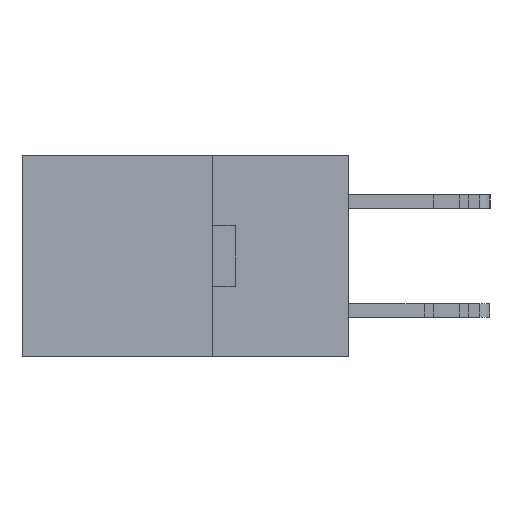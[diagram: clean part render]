
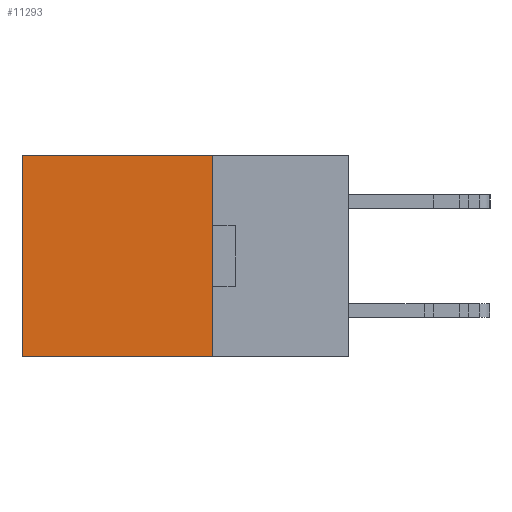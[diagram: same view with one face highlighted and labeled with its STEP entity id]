
A CAD part, left-side view. The second image highlights one B-rep face of the part: STEP entity #11293.
In plain terms, the highlighted planar face has unit normal (-1, 0, 0).
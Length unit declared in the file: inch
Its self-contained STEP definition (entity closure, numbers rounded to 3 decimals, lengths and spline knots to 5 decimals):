
#710 = DIRECTION ( 'NONE',  ( 0., 0., -1. ) ) ;
#2397 = AXIS2_PLACEMENT_3D ( 'NONE', #27128, #20479, #710 ) ;
#2577 = EDGE_CURVE ( 'NONE', #8262, #10466, #20778, .T. ) ;
#2801 = CARTESIAN_POINT ( 'NONE',  ( 0.2615, 0.25, -0.37 ) ) ;
#3636 = CARTESIAN_POINT ( 'NONE',  ( 0.2615, 0.6, 0. ) ) ;
#4208 = ORIENTED_EDGE ( 'NONE', *, *, #15069, .T. ) ;
#4857 = LINE ( 'NONE', #9745, #5923 ) ;
#5923 = VECTOR ( 'NONE', #20699, 39.37008 ) ;
#6328 = ORIENTED_EDGE ( 'NONE', *, *, #2577, .F. ) ;
#6806 = LINE ( 'NONE', #17851, #27389 ) ;
#7150 = VECTOR ( 'NONE', #16238, 39.37008 ) ;
#7528 = CARTESIAN_POINT ( 'NONE',  ( 0.2615, 0.25, -0.37 ) ) ;
#8262 = VERTEX_POINT ( 'NONE', #2801 ) ;
#8818 = EDGE_CURVE ( 'NONE', #19410, #8262, #27438, .T. ) ;
#9376 = FACE_OUTER_BOUND ( 'NONE', #19282, .T. ) ;
#9745 = CARTESIAN_POINT ( 'NONE',  ( 0.2615, 0.25, 0. ) ) ;
#10466 = VERTEX_POINT ( 'NONE', #16189 ) ;
#11204 = ORIENTED_EDGE ( 'NONE', *, *, #8818, .F. ) ;
#11293 = ADVANCED_FACE ( 'NONE', ( #9376 ), #18279, .F. ) ;
#15069 = EDGE_CURVE ( 'NONE', #20377, #10466, #6806, .T. ) ;
#16189 = CARTESIAN_POINT ( 'NONE',  ( 0.2615, 0.6, -0.37 ) ) ;
#16238 = DIRECTION ( 'NONE',  ( 0., 1., 0. ) ) ;
#16381 = DIRECTION ( 'NONE',  ( 0., 0., -1. ) ) ;
#17851 = CARTESIAN_POINT ( 'NONE',  ( 0.2615, 0.6, -0.37 ) ) ;
#18279 = PLANE ( 'NONE',  #2397 ) ;
#19282 = EDGE_LOOP ( 'NONE', ( #4208, #6328, #11204, #24480 ) ) ;
#19410 = VERTEX_POINT ( 'NONE', #19590 ) ;
#19590 = CARTESIAN_POINT ( 'NONE',  ( 0.2615, 0.25, 0. ) ) ;
#20377 = VERTEX_POINT ( 'NONE', #3636 ) ;
#20479 = DIRECTION ( 'NONE',  ( 1., 0., 0. ) ) ;
#20699 = DIRECTION ( 'NONE',  ( 0., 1., 0. ) ) ;
#20778 = LINE ( 'NONE', #22371, #7150 ) ;
#22371 = CARTESIAN_POINT ( 'NONE',  ( 0.2615, 0.25, -0.37 ) ) ;
#22800 = DIRECTION ( 'NONE',  ( 0., 0., -1. ) ) ;
#24058 = VECTOR ( 'NONE', #16381, 39.37008 ) ;
#24480 = ORIENTED_EDGE ( 'NONE', *, *, #27353, .T. ) ;
#27128 = CARTESIAN_POINT ( 'NONE',  ( 0.2615, 0.25, -0.37 ) ) ;
#27353 = EDGE_CURVE ( 'NONE', #19410, #20377, #4857, .T. ) ;
#27389 = VECTOR ( 'NONE', #22800, 39.37008 ) ;
#27438 = LINE ( 'NONE', #7528, #24058 ) ;
